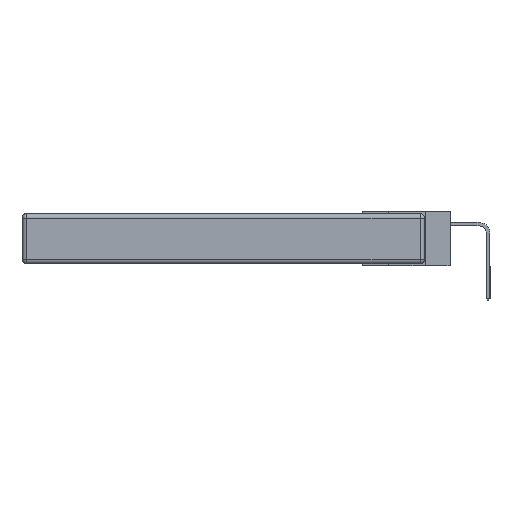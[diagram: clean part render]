
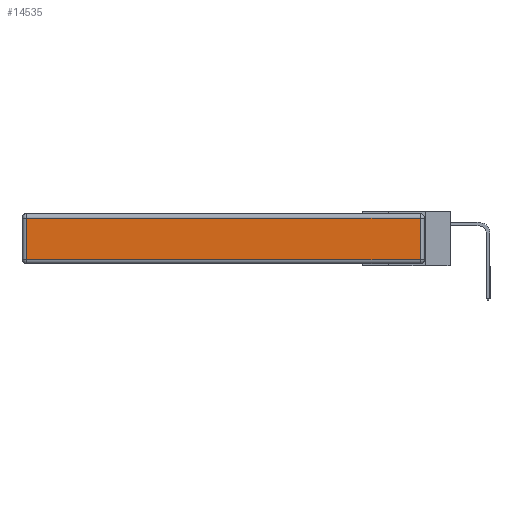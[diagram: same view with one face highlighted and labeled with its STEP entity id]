
A CAD part, left-side view. The second image highlights one B-rep face of the part: STEP entity #14535.
In plain terms, the highlighted planar face has unit normal (-1, 0, 0).
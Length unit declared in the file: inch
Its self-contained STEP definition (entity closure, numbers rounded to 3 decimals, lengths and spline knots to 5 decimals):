
#290 = PLANE ( 'NONE',  #3779 ) ;
#588 = ORIENTED_EDGE ( 'NONE', *, *, #13260, .T. ) ;
#876 = VECTOR ( 'NONE', #12857, 39.37008 ) ;
#1183 = CARTESIAN_POINT ( 'NONE',  ( 0., 0.03, -0.03 ) ) ;
#1365 = DIRECTION ( 'NONE',  ( 0., 0., 1. ) ) ;
#1840 = VECTOR ( 'NONE', #15329, 39.37008 ) ;
#2275 = CARTESIAN_POINT ( 'NONE',  ( 0., 2.72, -0.313 ) ) ;
#2304 = VERTEX_POINT ( 'NONE', #15919 ) ;
#2316 = EDGE_CURVE ( 'NONE', #2304, #13257, #5573, .T. ) ;
#2465 = FACE_OUTER_BOUND ( 'NONE', #2792, .T. ) ;
#2792 = EDGE_LOOP ( 'NONE', ( #588, #14203, #5555, #6907 ) ) ;
#3779 = AXIS2_PLACEMENT_3D ( 'NONE', #8255, #6994, #5680 ) ;
#4967 = CARTESIAN_POINT ( 'NONE',  ( 0., 2.72, -0.343 ) ) ;
#5555 = ORIENTED_EDGE ( 'NONE', *, *, #10002, .T. ) ;
#5573 = LINE ( 'NONE', #16037, #12590 ) ;
#5680 = DIRECTION ( 'NONE',  ( 0., 0., 1. ) ) ;
#6378 = VERTEX_POINT ( 'NONE', #12408 ) ;
#6472 = VERTEX_POINT ( 'NONE', #2275 ) ;
#6875 = CARTESIAN_POINT ( 'NONE',  ( 0., 2.75, -0.03 ) ) ;
#6907 = ORIENTED_EDGE ( 'NONE', *, *, #12183, .T. ) ;
#6994 = DIRECTION ( 'NONE',  ( -1., 0., 0. ) ) ;
#7761 = DIRECTION ( 'NONE',  ( 0., -1., 0. ) ) ;
#7887 = LINE ( 'NONE', #6875, #876 ) ;
#8255 = CARTESIAN_POINT ( 'NONE',  ( 0., 0., -0.343 ) ) ;
#10002 = EDGE_CURVE ( 'NONE', #13257, #6378, #7887, .T. ) ;
#12183 = EDGE_CURVE ( 'NONE', #6378, #6472, #17027, .T. ) ;
#12408 = CARTESIAN_POINT ( 'NONE',  ( 0., 2.72, -0.03 ) ) ;
#12590 = VECTOR ( 'NONE', #1365, 39.37008 ) ;
#12608 = LINE ( 'NONE', #14327, #13437 ) ;
#12857 = DIRECTION ( 'NONE',  ( 0., 1., 0. ) ) ;
#13257 = VERTEX_POINT ( 'NONE', #1183 ) ;
#13260 = EDGE_CURVE ( 'NONE', #6472, #2304, #12608, .T. ) ;
#13437 = VECTOR ( 'NONE', #7761, 39.37008 ) ;
#14203 = ORIENTED_EDGE ( 'NONE', *, *, #2316, .T. ) ;
#14327 = CARTESIAN_POINT ( 'NONE',  ( 0., 0., -0.313 ) ) ;
#14535 = ADVANCED_FACE ( 'NONE', ( #2465 ), #290, .T. ) ;
#15329 = DIRECTION ( 'NONE',  ( 0., 0., -1. ) ) ;
#15919 = CARTESIAN_POINT ( 'NONE',  ( 0., 0.03, -0.313 ) ) ;
#16037 = CARTESIAN_POINT ( 'NONE',  ( 0., 0.03, -0.343 ) ) ;
#17027 = LINE ( 'NONE', #4967, #1840 ) ;
